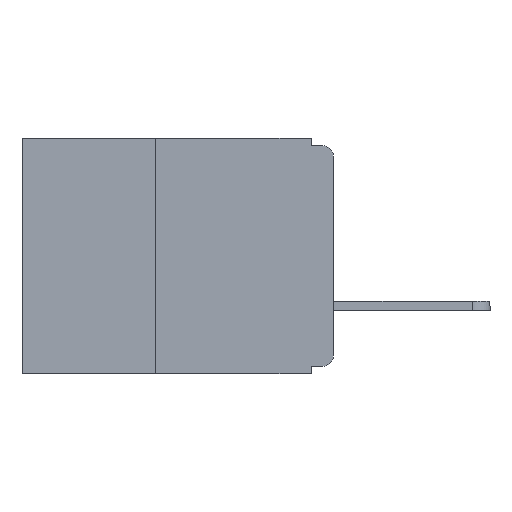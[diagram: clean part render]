
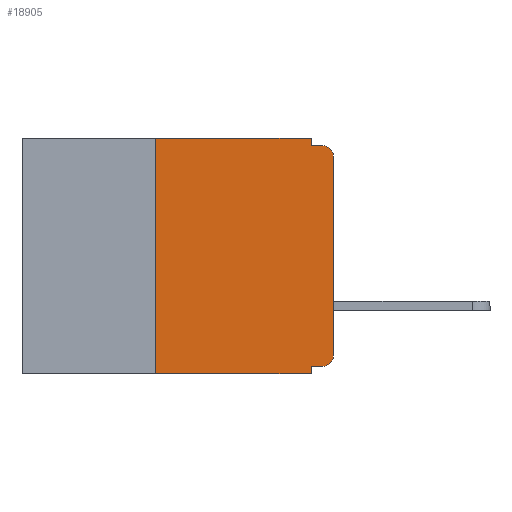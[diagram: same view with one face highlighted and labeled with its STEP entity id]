
A CAD part, left-side view. The second image highlights one B-rep face of the part: STEP entity #18905.
In plain terms, the highlighted planar face has unit normal (-1, 0, 0).
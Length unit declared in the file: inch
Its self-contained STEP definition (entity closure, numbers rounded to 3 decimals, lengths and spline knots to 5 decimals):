
#279 = CARTESIAN_POINT ( 'NONE',  ( 0., 0.437, 0. ) ) ;
#432 = LINE ( 'NONE', #1097, #10883 ) ;
#614 = VERTEX_POINT ( 'NONE', #22966 ) ;
#654 = VERTEX_POINT ( 'NONE', #22384 ) ;
#923 = DIRECTION ( 'NONE',  ( -1., 0., 0. ) ) ;
#1097 = CARTESIAN_POINT ( 'NONE',  ( 0., 0.031, 0. ) ) ;
#1170 = DIRECTION ( 'NONE',  ( 0., 0., 1. ) ) ;
#1260 = CARTESIAN_POINT ( 'NONE',  ( 0., 0.25, -0.33 ) ) ;
#1605 = CARTESIAN_POINT ( 'NONE',  ( 0., 0., -0.025 ) ) ;
#1951 = ORIENTED_EDGE ( 'NONE', *, *, #9029, .F. ) ;
#2300 = ORIENTED_EDGE ( 'NONE', *, *, #6637, .F. ) ;
#3048 = EDGE_CURVE ( 'NONE', #654, #3468, #8734, .T. ) ;
#3081 = DIRECTION ( 'NONE',  ( 0., 0., -1. ) ) ;
#3223 = ORIENTED_EDGE ( 'NONE', *, *, #20906, .F. ) ;
#3468 = VERTEX_POINT ( 'NONE', #16367 ) ;
#3840 = DIRECTION ( 'NONE',  ( 0., -1., 0. ) ) ;
#4203 = VERTEX_POINT ( 'NONE', #5604 ) ;
#4487 = EDGE_CURVE ( 'NONE', #16251, #17405, #5327, .T. ) ;
#5168 = CARTESIAN_POINT ( 'NONE',  ( 0., 0.031, 0. ) ) ;
#5217 = VERTEX_POINT ( 'NONE', #13373 ) ;
#5220 = DIRECTION ( 'NONE',  ( 0., -1., 0. ) ) ;
#5324 = AXIS2_PLACEMENT_3D ( 'NONE', #18909, #6626, #20953 ) ;
#5327 = LINE ( 'NONE', #17289, #16302 ) ;
#5391 = CARTESIAN_POINT ( 'NONE',  ( 0., 0.031, -0.33 ) ) ;
#5518 = EDGE_CURVE ( 'NONE', #654, #4203, #21937, .T. ) ;
#5578 = VECTOR ( 'NONE', #5220, 39.37008 ) ;
#5604 = CARTESIAN_POINT ( 'NONE',  ( 0., 0.031, -0.33 ) ) ;
#6539 = CARTESIAN_POINT ( 'NONE',  ( 0., 0.437, -0.33 ) ) ;
#6626 = DIRECTION ( 'NONE',  ( -1., 0., 0. ) ) ;
#6637 = EDGE_CURVE ( 'NONE', #5217, #4203, #25539, .T. ) ;
#7194 = ORIENTED_EDGE ( 'NONE', *, *, #5518, .T. ) ;
#7521 = DIRECTION ( 'NONE',  ( 0., 0., -1. ) ) ;
#8065 = VECTOR ( 'NONE', #1170, 39.37008 ) ;
#8075 = DIRECTION ( 'NONE',  ( 0., 1., 0. ) ) ;
#8290 = AXIS2_PLACEMENT_3D ( 'NONE', #279, #10770, #24878 ) ;
#8610 = PLANE ( 'NONE',  #8290 ) ;
#8734 = LINE ( 'NONE', #1260, #8065 ) ;
#9029 = EDGE_CURVE ( 'NONE', #11041, #22058, #432, .T. ) ;
#9251 = VECTOR ( 'NONE', #3840, 39.37008 ) ;
#9474 = VECTOR ( 'NONE', #11429, 39.37008 ) ;
#9503 = CARTESIAN_POINT ( 'NONE',  ( 0., 0.031, -0.01 ) ) ;
#10174 = CARTESIAN_POINT ( 'NONE',  ( 0., 0., -0.32 ) ) ;
#10770 = DIRECTION ( 'NONE',  ( 1., 0., 0. ) ) ;
#10883 = VECTOR ( 'NONE', #3081, 39.37008 ) ;
#11041 = VERTEX_POINT ( 'NONE', #5168 ) ;
#11332 = VECTOR ( 'NONE', #7521, 39.37008 ) ;
#11429 = DIRECTION ( 'NONE',  ( 0., -1., 0. ) ) ;
#12358 = ORIENTED_EDGE ( 'NONE', *, *, #12901, .F. ) ;
#12444 = CARTESIAN_POINT ( 'NONE',  ( 0., 0.015, -0.32 ) ) ;
#12901 = EDGE_CURVE ( 'NONE', #22058, #614, #16574, .T. ) ;
#13168 = VECTOR ( 'NONE', #8075, 39.37008 ) ;
#13344 = CARTESIAN_POINT ( 'NONE',  ( 0., 0.015, -0.305 ) ) ;
#13373 = CARTESIAN_POINT ( 'NONE',  ( 0., 0.031, -0.32 ) ) ;
#14076 = VERTEX_POINT ( 'NONE', #12444 ) ;
#14226 = AXIS2_PLACEMENT_3D ( 'NONE', #13344, #923, #15374 ) ;
#14337 = CARTESIAN_POINT ( 'NONE',  ( 0., 0., -0.305 ) ) ;
#15374 = DIRECTION ( 'NONE',  ( 0., 0., -1. ) ) ;
#16251 = VERTEX_POINT ( 'NONE', #14337 ) ;
#16302 = VECTOR ( 'NONE', #17295, 39.37008 ) ;
#16367 = CARTESIAN_POINT ( 'NONE',  ( 0., 0.25, 0. ) ) ;
#16547 = EDGE_CURVE ( 'NONE', #14076, #16251, #23336, .T. ) ;
#16574 = LINE ( 'NONE', #18261, #9251 ) ;
#17289 = CARTESIAN_POINT ( 'NONE',  ( 0., 0., 0. ) ) ;
#17295 = DIRECTION ( 'NONE',  ( 0., 0., 1. ) ) ;
#17405 = VERTEX_POINT ( 'NONE', #1605 ) ;
#17763 = ORIENTED_EDGE ( 'NONE', *, *, #16547, .T. ) ;
#18261 = CARTESIAN_POINT ( 'NONE',  ( 0., 0., -0.01 ) ) ;
#18582 = LINE ( 'NONE', #10174, #13168 ) ;
#18905 = ADVANCED_FACE ( 'NONE', ( #22269 ), #8610, .F. ) ;
#18909 = CARTESIAN_POINT ( 'NONE',  ( 0., 0.015, -0.025 ) ) ;
#19367 = ORIENTED_EDGE ( 'NONE', *, *, #22887, .F. ) ;
#19420 = EDGE_LOOP ( 'NONE', ( #24659, #20620, #12358, #1951, #3223, #25617, #7194, #2300, #19367, #17763 ) ) ;
#19652 = LINE ( 'NONE', #23540, #9474 ) ;
#20620 = ORIENTED_EDGE ( 'NONE', *, *, #24914, .T. ) ;
#20906 = EDGE_CURVE ( 'NONE', #3468, #11041, #19652, .T. ) ;
#20953 = DIRECTION ( 'NONE',  ( 0., 0., -1. ) ) ;
#21937 = LINE ( 'NONE', #6539, #5578 ) ;
#22058 = VERTEX_POINT ( 'NONE', #9503 ) ;
#22269 = FACE_OUTER_BOUND ( 'NONE', #19420, .T. ) ;
#22384 = CARTESIAN_POINT ( 'NONE',  ( 0., 0.25, -0.33 ) ) ;
#22887 = EDGE_CURVE ( 'NONE', #14076, #5217, #18582, .T. ) ;
#22966 = CARTESIAN_POINT ( 'NONE',  ( 0., 0.015, -0.01 ) ) ;
#23336 = CIRCLE ( 'NONE', #14226, 0.015 ) ;
#23540 = CARTESIAN_POINT ( 'NONE',  ( 0., 0.437, 0. ) ) ;
#24659 = ORIENTED_EDGE ( 'NONE', *, *, #4487, .T. ) ;
#24878 = DIRECTION ( 'NONE',  ( 0., 0., -1. ) ) ;
#24914 = EDGE_CURVE ( 'NONE', #17405, #614, #26487, .T. ) ;
#25539 = LINE ( 'NONE', #5391, #11332 ) ;
#25617 = ORIENTED_EDGE ( 'NONE', *, *, #3048, .F. ) ;
#26487 = CIRCLE ( 'NONE', #5324, 0.015 ) ;
